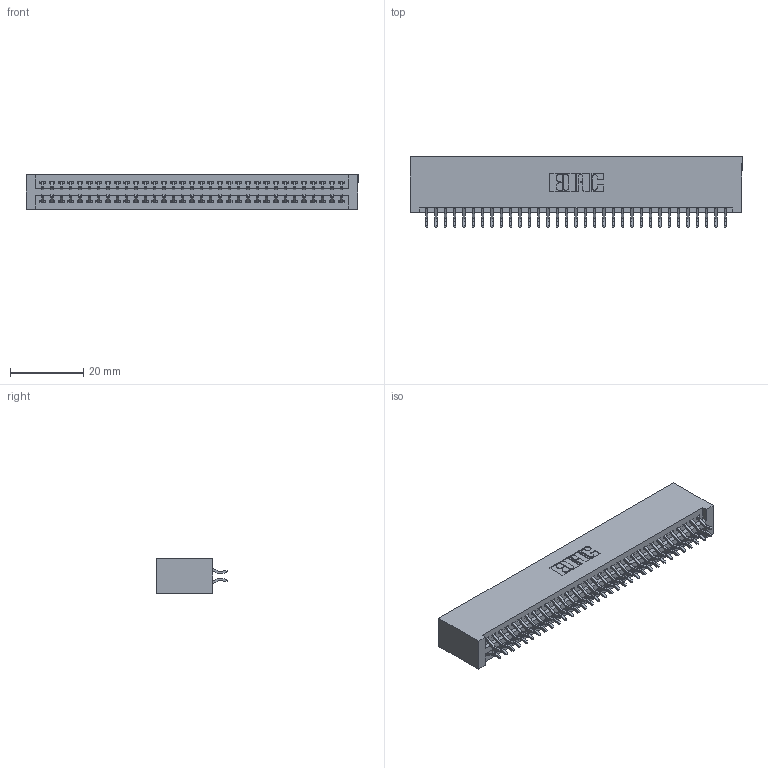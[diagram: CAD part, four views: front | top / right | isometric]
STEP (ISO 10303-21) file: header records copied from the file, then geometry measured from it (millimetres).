
FILE_DESCRIPTION (( 'STEP AP203' ), '1' );
FILE_NAME ('345-066-556-201.STEP', '2018-09-28T23:24:24', ( '' ), ( '' ), 'SwSTEP 2.0', 'SolidWorks 2016', '' );
FILE_SCHEMA (( 'CONFIG_CONTROL_DESIGN' ));
Length unit declared in the file: inch
Products named in the file (3): 345-066-556-201; 345 Part_No Mounting Lugs; 345-292-001_556 Tail
Assembly tree (67 placements, depth 2):
  345-066-556-201
    345 Part_No Mounting Lugs
    345-292-001_556 Tail  x66
Bounding box: 90.42 x 19.24 x 9.4 mm (x, y, z)
Volume: 9313.6 mm3; surface area: 13838.3 mm2
Topology: 67 solids, 67 shells, 3814 faces, 11339 edges, 7470 vertices
Faces by surface type: plane 2518, cylinder 1296
Entity records: 27047 total; most frequent: CARTESIAN_POINT 4556, ORIENTED_EDGE 4478, DIRECTION 4011, EDGE_CURVE 2239, LINE 1975, VECTOR 1975, VERTEX_POINT 1490, AXIS2_PLACEMENT_3D 1018
